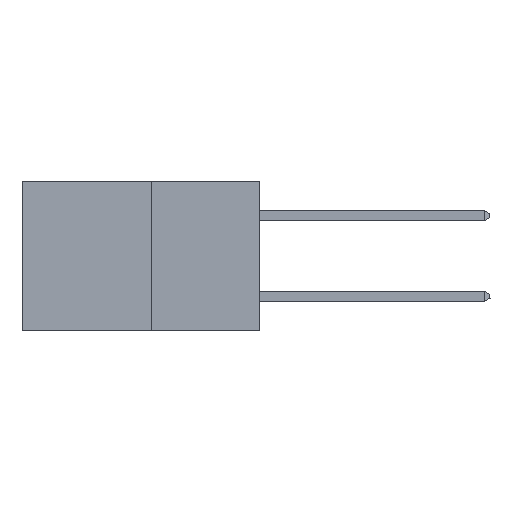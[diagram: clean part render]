
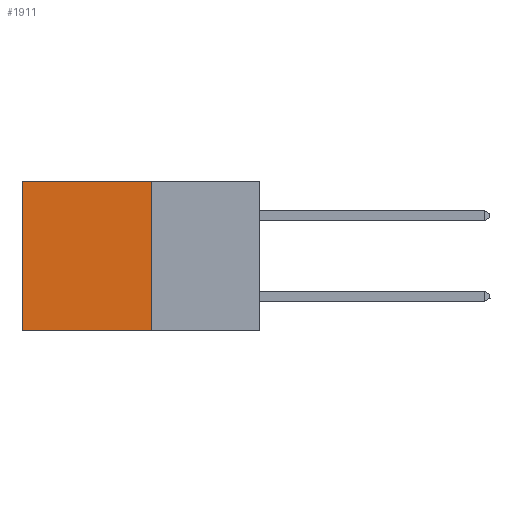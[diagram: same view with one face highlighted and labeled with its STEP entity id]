
A CAD part, left-side view. The second image highlights one B-rep face of the part: STEP entity #1911.
In plain terms, the highlighted planar face has unit normal (-1, 0, 0).
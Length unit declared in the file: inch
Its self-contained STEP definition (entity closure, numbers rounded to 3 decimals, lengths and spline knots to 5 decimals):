
#1061 = DIRECTION ( 'NONE',  ( 0., 0., -1. ) ) ;
#1361 = VERTEX_POINT ( 'NONE', #21944 ) ;
#1438 = VERTEX_POINT ( 'NONE', #17220 ) ;
#1527 = ORIENTED_EDGE ( 'NONE', *, *, #17789, .T. ) ;
#1835 = FACE_OUTER_BOUND ( 'NONE', #3466, .T. ) ;
#1911 = ADVANCED_FACE ( 'NONE', ( #1835 ), #2055, .F. ) ;
#1994 = CARTESIAN_POINT ( 'NONE',  ( 0.277, 0.27, -0.37 ) ) ;
#2055 = PLANE ( 'NONE',  #13960 ) ;
#2211 = CARTESIAN_POINT ( 'NONE',  ( 0.277, 0.27, 0. ) ) ;
#3466 = EDGE_LOOP ( 'NONE', ( #1527, #16726, #14592, #19699 ) ) ;
#6005 = CARTESIAN_POINT ( 'NONE',  ( 0.277, 0.27, 0. ) ) ;
#6160 = CARTESIAN_POINT ( 'NONE',  ( 0.277, 0.59, -0.37 ) ) ;
#6171 = VECTOR ( 'NONE', #17627, 39.37008 ) ;
#6702 = LINE ( 'NONE', #1994, #6171 ) ;
#7022 = EDGE_CURVE ( 'NONE', #18997, #1361, #6702, .T. ) ;
#7648 = VECTOR ( 'NONE', #13995, 39.37008 ) ;
#10468 = DIRECTION ( 'NONE',  ( 0., 0., -1. ) ) ;
#11148 = DIRECTION ( 'NONE',  ( 0., 1., 0. ) ) ;
#11385 = CARTESIAN_POINT ( 'NONE',  ( 0.277, 0.27, -0.37 ) ) ;
#12261 = LINE ( 'NONE', #19132, #7648 ) ;
#12484 = VECTOR ( 'NONE', #1061, 39.37008 ) ;
#13535 = LINE ( 'NONE', #6005, #17613 ) ;
#13960 = AXIS2_PLACEMENT_3D ( 'NONE', #11385, #14349, #10468 ) ;
#13995 = DIRECTION ( 'NONE',  ( 0., 1., 0. ) ) ;
#14349 = DIRECTION ( 'NONE',  ( 1., 0., 0. ) ) ;
#14592 = ORIENTED_EDGE ( 'NONE', *, *, #7022, .F. ) ;
#16687 = EDGE_CURVE ( 'NONE', #1361, #21490, #12261, .T. ) ;
#16726 = ORIENTED_EDGE ( 'NONE', *, *, #16687, .F. ) ;
#17106 = LINE ( 'NONE', #6160, #12484 ) ;
#17220 = CARTESIAN_POINT ( 'NONE',  ( 0.277, 0.59, 0. ) ) ;
#17613 = VECTOR ( 'NONE', #11148, 39.37008 ) ;
#17627 = DIRECTION ( 'NONE',  ( 0., 0., -1. ) ) ;
#17789 = EDGE_CURVE ( 'NONE', #1438, #21490, #17106, .T. ) ;
#18997 = VERTEX_POINT ( 'NONE', #2211 ) ;
#19132 = CARTESIAN_POINT ( 'NONE',  ( 0.277, 0.27, -0.37 ) ) ;
#19699 = ORIENTED_EDGE ( 'NONE', *, *, #19899, .T. ) ;
#19899 = EDGE_CURVE ( 'NONE', #18997, #1438, #13535, .T. ) ;
#20458 = CARTESIAN_POINT ( 'NONE',  ( 0.277, 0.59, -0.37 ) ) ;
#21490 = VERTEX_POINT ( 'NONE', #20458 ) ;
#21944 = CARTESIAN_POINT ( 'NONE',  ( 0.277, 0.27, -0.37 ) ) ;
